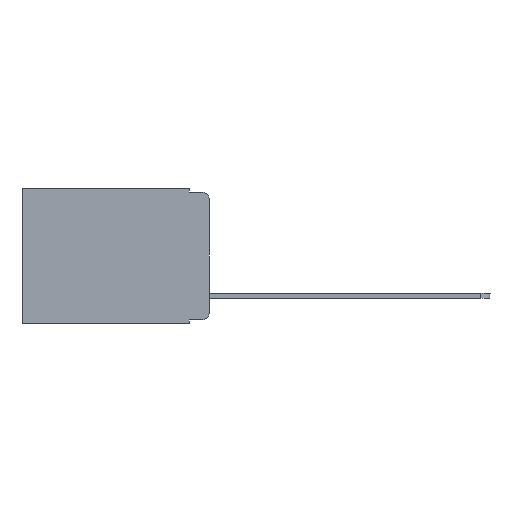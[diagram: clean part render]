
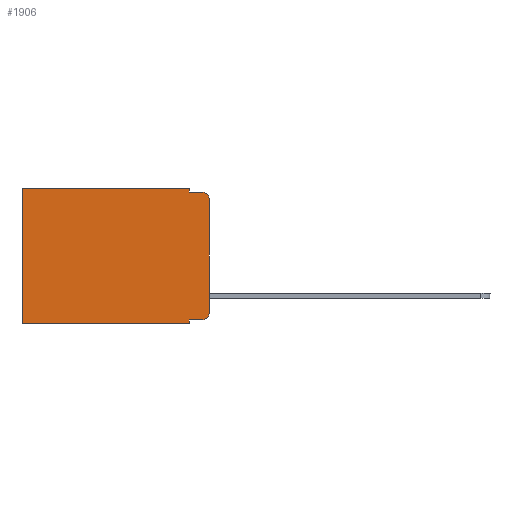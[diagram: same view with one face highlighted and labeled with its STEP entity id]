
A CAD part, left-side view. The second image highlights one B-rep face of the part: STEP entity #1906.
In plain terms, the highlighted planar face has unit normal (-1, 0, 0).
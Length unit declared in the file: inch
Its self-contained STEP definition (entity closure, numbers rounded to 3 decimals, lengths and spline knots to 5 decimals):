
#40 = CARTESIAN_POINT ( 'NONE',  ( 0.298, 0.02, -0.03 ) ) ;
#83 = AXIS2_PLACEMENT_3D ( 'NONE', #1858, #1037, #3924 ) ;
#235 = VERTEX_POINT ( 'NONE', #7835 ) ;
#427 = DIRECTION ( 'NONE',  ( 0., 0., -1. ) ) ;
#428 = ORIENTED_EDGE ( 'NONE', *, *, #2288, .F. ) ;
#556 = CARTESIAN_POINT ( 'NONE',  ( 0.298, 0.02, -0.333 ) ) ;
#673 = CARTESIAN_POINT ( 'NONE',  ( 0.298, 0.051, 0. ) ) ;
#878 = VERTEX_POINT ( 'NONE', #4118 ) ;
#922 = VERTEX_POINT ( 'NONE', #6889 ) ;
#1037 = DIRECTION ( 'NONE',  ( 1., 0., 0. ) ) ;
#1040 = EDGE_CURVE ( 'NONE', #922, #878, #4161, .T. ) ;
#1116 = LINE ( 'NONE', #2674, #1580 ) ;
#1202 = VECTOR ( 'NONE', #5533, 39.37008 ) ;
#1216 = ORIENTED_EDGE ( 'NONE', *, *, #8522, .T. ) ;
#1290 = DIRECTION ( 'NONE',  ( 0., 0., -1. ) ) ;
#1321 = VERTEX_POINT ( 'NONE', #7801 ) ;
#1521 = VECTOR ( 'NONE', #3473, 39.37008 ) ;
#1580 = VECTOR ( 'NONE', #427, 39.37008 ) ;
#1654 = ORIENTED_EDGE ( 'NONE', *, *, #5834, .T. ) ;
#1802 = ORIENTED_EDGE ( 'NONE', *, *, #8226, .F. ) ;
#1858 = CARTESIAN_POINT ( 'NONE',  ( 0.298, 0., 0. ) ) ;
#1906 = ADVANCED_FACE ( 'NONE', ( #8297 ), #7502, .F. ) ;
#1972 = DIRECTION ( 'NONE',  ( -1., 0., 0. ) ) ;
#2005 = CARTESIAN_POINT ( 'NONE',  ( 0.298, 0.051, -0.333 ) ) ;
#2089 = VERTEX_POINT ( 'NONE', #8009 ) ;
#2141 = EDGE_CURVE ( 'NONE', #2089, #4520, #1116, .T. ) ;
#2288 = EDGE_CURVE ( 'NONE', #922, #6495, #7848, .T. ) ;
#2329 = CARTESIAN_POINT ( 'NONE',  ( 0.298, 0.051, -0.343 ) ) ;
#2343 = EDGE_CURVE ( 'NONE', #6495, #3026, #5756, .T. ) ;
#2604 = CARTESIAN_POINT ( 'NONE',  ( 0.298, 0.02, -0.01 ) ) ;
#2627 = ORIENTED_EDGE ( 'NONE', *, *, #2343, .F. ) ;
#2674 = CARTESIAN_POINT ( 'NONE',  ( 0.298, 0., 0. ) ) ;
#2688 = CARTESIAN_POINT ( 'NONE',  ( 0.298, 0., 0. ) ) ;
#2751 = CARTESIAN_POINT ( 'NONE',  ( 0.298, 0.02, -0.313 ) ) ;
#2809 = CARTESIAN_POINT ( 'NONE',  ( 0.298, 0.051, -0.01 ) ) ;
#2821 = EDGE_CURVE ( 'NONE', #235, #6960, #7094, .T. ) ;
#2856 = DIRECTION ( 'NONE',  ( 0., 0., -1. ) ) ;
#2889 = CARTESIAN_POINT ( 'NONE',  ( 0.298, 0., -0.313 ) ) ;
#3026 = VERTEX_POINT ( 'NONE', #2604 ) ;
#3154 = EDGE_CURVE ( 'NONE', #8521, #4520, #6956, .T. ) ;
#3473 = DIRECTION ( 'NONE',  ( 0., -1., 0. ) ) ;
#3503 = DIRECTION ( 'NONE',  ( -1., 0., 0. ) ) ;
#3523 = DIRECTION ( 'NONE',  ( 0., -1., 0. ) ) ;
#3612 = VECTOR ( 'NONE', #4293, 39.37008 ) ;
#3732 = ORIENTED_EDGE ( 'NONE', *, *, #3154, .T. ) ;
#3784 = AXIS2_PLACEMENT_3D ( 'NONE', #2751, #3503, #1290 ) ;
#3924 = DIRECTION ( 'NONE',  ( 0., 0., -1. ) ) ;
#4118 = CARTESIAN_POINT ( 'NONE',  ( 0.298, 0.473, 0. ) ) ;
#4121 = EDGE_CURVE ( 'NONE', #2089, #3026, #5383, .T. ) ;
#4161 = LINE ( 'NONE', #2688, #1202 ) ;
#4229 = CARTESIAN_POINT ( 'NONE',  ( 0.298, 0.473, 0. ) ) ;
#4293 = DIRECTION ( 'NONE',  ( 0., 1., 0. ) ) ;
#4320 = DIRECTION ( 'NONE',  ( 0., 0., -1. ) ) ;
#4520 = VERTEX_POINT ( 'NONE', #2889 ) ;
#4567 = EDGE_LOOP ( 'NONE', ( #7525, #6033, #2627, #428, #7726, #1654, #1802, #4761, #1216, #3732 ) ) ;
#4761 = ORIENTED_EDGE ( 'NONE', *, *, #2821, .F. ) ;
#4802 = LINE ( 'NONE', #4229, #7033 ) ;
#5365 = VECTOR ( 'NONE', #3523, 39.37008 ) ;
#5383 = CIRCLE ( 'NONE', #7174, 0.02 ) ;
#5533 = DIRECTION ( 'NONE',  ( 0., 1., 0. ) ) ;
#5756 = LINE ( 'NONE', #2809, #5365 ) ;
#5834 = EDGE_CURVE ( 'NONE', #878, #1321, #4802, .T. ) ;
#6033 = ORIENTED_EDGE ( 'NONE', *, *, #4121, .T. ) ;
#6315 = LINE ( 'NONE', #2005, #1521 ) ;
#6495 = VERTEX_POINT ( 'NONE', #7908 ) ;
#6889 = CARTESIAN_POINT ( 'NONE',  ( 0.298, 0.051, 0. ) ) ;
#6956 = CIRCLE ( 'NONE', #3784, 0.02 ) ;
#6960 = VERTEX_POINT ( 'NONE', #2329 ) ;
#7033 = VECTOR ( 'NONE', #7792, 39.37008 ) ;
#7094 = LINE ( 'NONE', #673, #7290 ) ;
#7174 = AXIS2_PLACEMENT_3D ( 'NONE', #40, #1972, #4320 ) ;
#7286 = CARTESIAN_POINT ( 'NONE',  ( 0.298, 0., -0.343 ) ) ;
#7290 = VECTOR ( 'NONE', #7745, 39.37008 ) ;
#7300 = VECTOR ( 'NONE', #2856, 39.37008 ) ;
#7502 = PLANE ( 'NONE',  #83 ) ;
#7525 = ORIENTED_EDGE ( 'NONE', *, *, #2141, .F. ) ;
#7726 = ORIENTED_EDGE ( 'NONE', *, *, #1040, .T. ) ;
#7745 = DIRECTION ( 'NONE',  ( 0., 0., -1. ) ) ;
#7792 = DIRECTION ( 'NONE',  ( 0., 0., -1. ) ) ;
#7801 = CARTESIAN_POINT ( 'NONE',  ( 0.298, 0.473, -0.343 ) ) ;
#7835 = CARTESIAN_POINT ( 'NONE',  ( 0.298, 0.051, -0.333 ) ) ;
#7848 = LINE ( 'NONE', #9246, #7300 ) ;
#7854 = LINE ( 'NONE', #7286, #3612 ) ;
#7908 = CARTESIAN_POINT ( 'NONE',  ( 0.298, 0.051, -0.01 ) ) ;
#8009 = CARTESIAN_POINT ( 'NONE',  ( 0.298, 0., -0.03 ) ) ;
#8226 = EDGE_CURVE ( 'NONE', #6960, #1321, #7854, .T. ) ;
#8297 = FACE_OUTER_BOUND ( 'NONE', #4567, .T. ) ;
#8521 = VERTEX_POINT ( 'NONE', #556 ) ;
#8522 = EDGE_CURVE ( 'NONE', #235, #8521, #6315, .T. ) ;
#9246 = CARTESIAN_POINT ( 'NONE',  ( 0.298, 0.051, 0. ) ) ;
